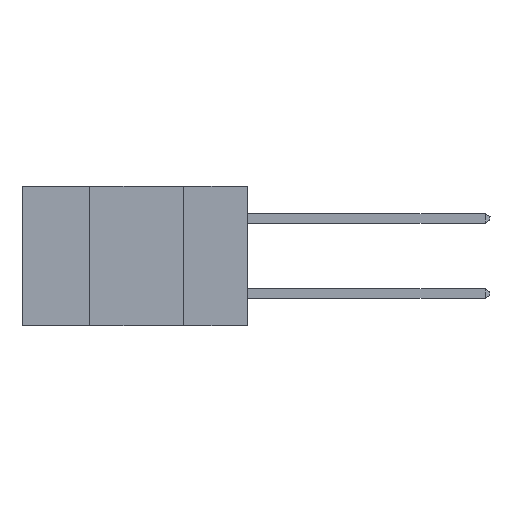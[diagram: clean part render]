
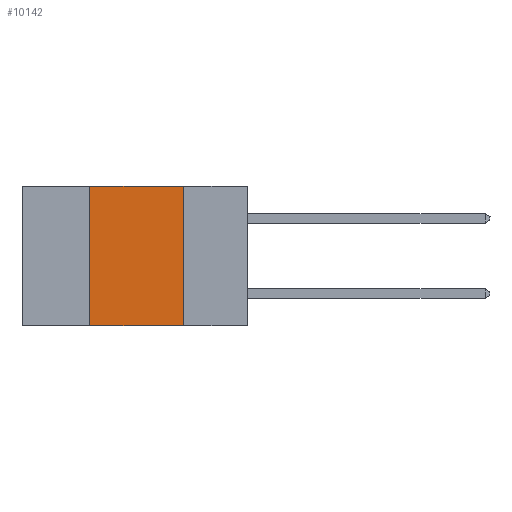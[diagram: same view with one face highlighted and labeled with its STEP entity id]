
A CAD part, left-side view. The second image highlights one B-rep face of the part: STEP entity #10142.
In plain terms, the highlighted planar face has unit normal (-1, 0, 0).
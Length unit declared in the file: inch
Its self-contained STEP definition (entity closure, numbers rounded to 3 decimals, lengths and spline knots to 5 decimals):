
#1342 = CARTESIAN_POINT ( 'NONE',  ( 0., 0.6, 0. ) ) ;
#1384 = DIRECTION ( 'NONE',  ( 0., -1., 0. ) ) ;
#2643 = EDGE_LOOP ( 'NONE', ( #18606, #21026, #19276, #4962 ) ) ;
#3193 = LINE ( 'NONE', #14334, #21238 ) ;
#3276 = DIRECTION ( 'NONE',  ( 0., -1., 0. ) ) ;
#4807 = FACE_OUTER_BOUND ( 'NONE', #2643, .T. ) ;
#4962 = ORIENTED_EDGE ( 'NONE', *, *, #21860, .T. ) ;
#6156 = VECTOR ( 'NONE', #1384, 39.37008 ) ;
#6470 = DIRECTION ( 'NONE',  ( 0., 0., -1. ) ) ;
#6538 = CARTESIAN_POINT ( 'NONE',  ( 0., 0.17, 0. ) ) ;
#6867 = VERTEX_POINT ( 'NONE', #10880 ) ;
#6892 = DIRECTION ( 'NONE',  ( 0., 0., -1. ) ) ;
#7347 = CARTESIAN_POINT ( 'NONE',  ( 0., 0.17, -0.37 ) ) ;
#7793 = EDGE_CURVE ( 'NONE', #7911, #12452, #16210, .T. ) ;
#7911 = VERTEX_POINT ( 'NONE', #16448 ) ;
#9968 = EDGE_CURVE ( 'NONE', #6867, #7911, #11177, .T. ) ;
#10142 = ADVANCED_FACE ( 'NONE', ( #4807 ), #22854, .F. ) ;
#10294 = VECTOR ( 'NONE', #3276, 39.37008 ) ;
#10880 = CARTESIAN_POINT ( 'NONE',  ( 0., 0.42, -0.37 ) ) ;
#11177 = LINE ( 'NONE', #11291, #11552 ) ;
#11291 = CARTESIAN_POINT ( 'NONE',  ( 0., 0.42, -0.37 ) ) ;
#11552 = VECTOR ( 'NONE', #18591, 39.37008 ) ;
#12370 = CARTESIAN_POINT ( 'NONE',  ( 0., 0.6, 0. ) ) ;
#12452 = VERTEX_POINT ( 'NONE', #6538 ) ;
#14334 = CARTESIAN_POINT ( 'NONE',  ( 0., 0.17, -0.37 ) ) ;
#15579 = DIRECTION ( 'NONE',  ( 1., 0., 0. ) ) ;
#15857 = LINE ( 'NONE', #22898, #6156 ) ;
#16160 = EDGE_CURVE ( 'NONE', #12452, #21982, #3193, .T. ) ;
#16210 = LINE ( 'NONE', #12370, #10294 ) ;
#16448 = CARTESIAN_POINT ( 'NONE',  ( 0., 0.42, 0. ) ) ;
#18591 = DIRECTION ( 'NONE',  ( 0., 0., 1. ) ) ;
#18606 = ORIENTED_EDGE ( 'NONE', *, *, #16160, .F. ) ;
#19276 = ORIENTED_EDGE ( 'NONE', *, *, #9968, .F. ) ;
#21026 = ORIENTED_EDGE ( 'NONE', *, *, #7793, .F. ) ;
#21238 = VECTOR ( 'NONE', #6892, 39.37008 ) ;
#21860 = EDGE_CURVE ( 'NONE', #6867, #21982, #15857, .T. ) ;
#21982 = VERTEX_POINT ( 'NONE', #7347 ) ;
#22854 = PLANE ( 'NONE',  #23367 ) ;
#22898 = CARTESIAN_POINT ( 'NONE',  ( 0., 0.6, -0.37 ) ) ;
#23367 = AXIS2_PLACEMENT_3D ( 'NONE', #1342, #15579, #6470 ) ;
